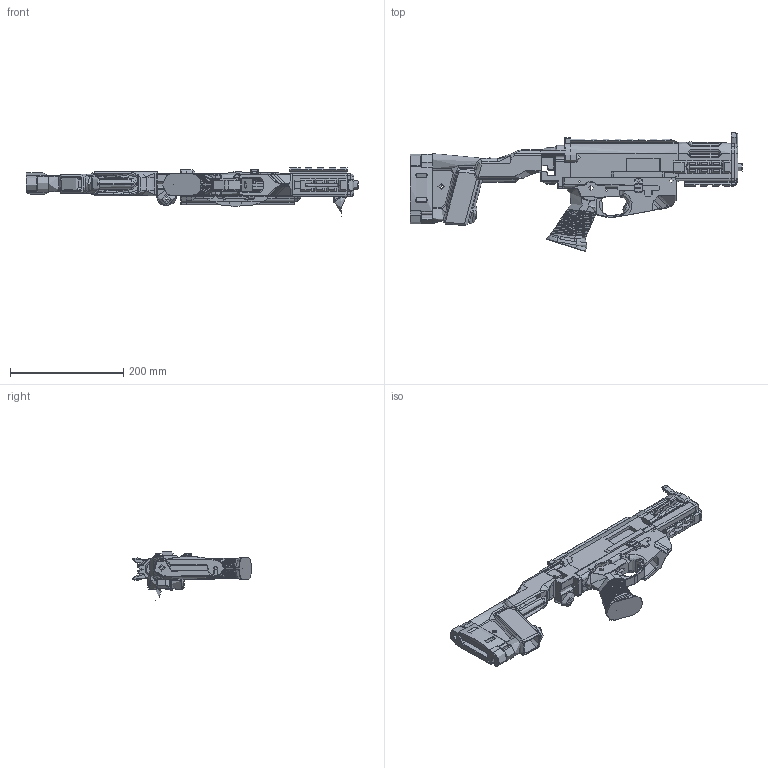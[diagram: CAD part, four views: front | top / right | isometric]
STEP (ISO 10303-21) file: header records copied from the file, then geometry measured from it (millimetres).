
FILE_DESCRIPTION(/* description */ ('','CAx-IF Rec.Pracs.---Representation and Presentation of Product Manufacturing Information (PMI)---3.8---2014-02-18'),/* implementation_level */ '2;1');
FILE_NAME(/* name */ 'WTF-9MV Full Assembly V1.2.stp',/* time_stamp */ '2020-05-13T19:39:10-07:00',/* author */ ('Uber Lobster'),/* organization */ (''),/* preprocessor_version */ 'ST-DEVELOPER v16.13',/* originating_system */ 'Autodesk Inventor 2018',/* authorisation */ '');
FILE_SCHEMA (('AP242_MANAGED_MODEL_BASED_3D_ENGINEERING_MIM_LF { 1 0 10303 442 1 1 4 }'));
Products named in the file (35): WTF-9MV; WTF-9MV_bolt_housing; WTF9 V1 FINAL_11; WTF-9MV_charging_handle; WTF-9MV_ejector; WTF9 V1 FINAL_15; WTF-9MV_ejector_mount; WTF9 V1 FINAL_8; WTF-9MV_upper_receiver; WTF9 V1 FINAL_9; WTF-9MV_pistol_grip; WTF-9MV_feed_ramp; WTF9 V1 FINAL; WTF-9MV_lower_receiver; WTF-9MV_mag_catch; WTF-9MV_mag_catch_mount; WTF9 V1 FINAL_7; WTF-9MV_mag_catch_rod; WTF9 V1 FINAL_20; WTF-9H_mag_release_pivot_pin; WTF-9MV_rear_end_cap; WTF9 V1 FINAL_6; WTF-9MV_stock; WTF9 V1 FINAL_21; WTF-9MV_stock_brace_1; WTF9 V1 FINAL_18; WTF-9MV_stock_brace_2; WTF9 V1 FINAL_14; WTF-9MV_stock_lock; WTF9 V1 FINAL_2; Glock 9mm long barrel; Lower Bolt; Upper bolt; WTF9MV_barrel_retainer_cap; WTF9MV_barrel_retainer_grip
Assembly tree (34 placements, depth 3):
  WTF-9MV
    WTF-9MV_bolt_housing
      WTF9 V1 FINAL_11
    WTF-9MV_charging_handle
    WTF-9MV_ejector
      WTF9 V1 FINAL_15
    WTF-9MV_ejector_mount
      WTF9 V1 FINAL_8
    WTF-9MV_upper_receiver
      WTF9 V1 FINAL_9
    WTF-9MV_pistol_grip
    WTF-9MV_feed_ramp
      WTF9 V1 FINAL
    WTF-9MV_lower_receiver
    WTF-9MV_mag_catch
    WTF-9MV_mag_catch_mount
      WTF9 V1 FINAL_7
    WTF-9MV_mag_catch_rod
      WTF9 V1 FINAL_20
    WTF-9H_mag_release_pivot_pin
    WTF-9MV_rear_end_cap
      WTF9 V1 FINAL_6
    WTF-9MV_stock
      WTF9 V1 FINAL_21
    WTF-9MV_stock_brace_1
      WTF9 V1 FINAL_18
    WTF-9MV_stock_brace_2
      WTF9 V1 FINAL_14
    WTF-9MV_stock_lock
      WTF9 V1 FINAL_2
    Glock 9mm long barrel
    Lower Bolt
    Upper bolt
    WTF9MV_barrel_retainer_cap
    WTF9MV_barrel_retainer_grip
Bounding box: 586.63 x 210.17 x 84.88 mm (x, y, z)
Volume: 1166443.1 mm3
Topology: 22 solids, 31 shells, 3111 faces, 8193 edges, 5090 vertices
Faces by surface type: plane 1392, bspline 724, cylinder 695, torus 165, cone 96, sphere 39
Full cylindrical faces by diameter (mm): 1 x2, 1.7 x1, 2 x1, 2.2 x1, 2.4 x5, 2.5 x4, 2.6 x2, 2.968 x2, 3 x2, 3.175 x4, 3.469 x4, 3.5 x3, 3.566 x1, 3.962 x1, 4 x4, 4.1 x3, 4.5 x7, 5.105 x1, 5.346 x1, 5.4 x2, 5.5 x2, 5.8 x1, 5.9 x1, 6 x2, 6.2 x1, 6.34 x1, 6.375 x1, 6.4 x2, 7.8 x1, 8 x2
Entity records: 153360 total; most frequent: CARTESIAN_POINT 78289, ORIENTED_EDGE 15816, DIRECTION 13771, EDGE_CURVE 7902, VERTEX_POINT 5010, AXIS2_PLACEMENT_3D 4723, LINE 4501, VECTOR 4501
